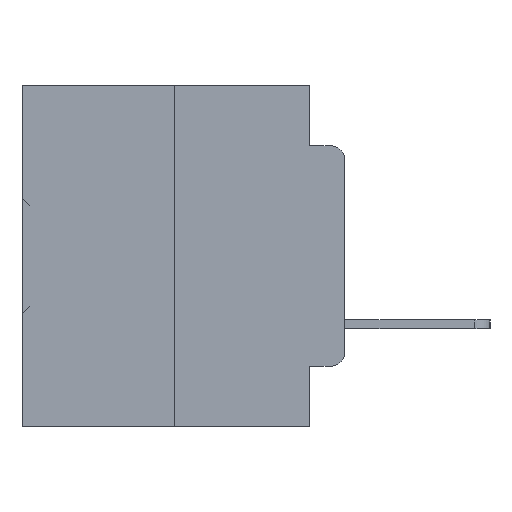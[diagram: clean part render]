
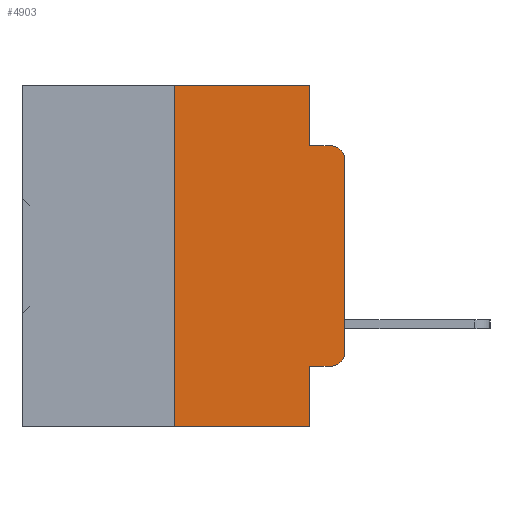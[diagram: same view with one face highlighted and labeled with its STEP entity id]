
A CAD part, left-side view. The second image highlights one B-rep face of the part: STEP entity #4903.
In plain terms, the highlighted planar face has unit normal (-1, 0, 0).
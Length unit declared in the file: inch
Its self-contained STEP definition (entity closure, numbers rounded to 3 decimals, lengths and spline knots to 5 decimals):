
#612 = DIRECTION ( 'NONE',  ( -1., 0., 0. ) ) ;
#797 = VERTEX_POINT ( 'NONE', #19545 ) ;
#963 = CIRCLE ( 'NONE', #14229, 0.02 ) ;
#1004 = CARTESIAN_POINT ( 'NONE',  ( 0., 0.051, -0.5 ) ) ;
#1061 = CARTESIAN_POINT ( 'NONE',  ( 0., 0.02, -0.1085 ) ) ;
#1221 = CARTESIAN_POINT ( 'NONE',  ( 0., 0.051, 0. ) ) ;
#2265 = LINE ( 'NONE', #32756, #8980 ) ;
#3630 = DIRECTION ( 'NONE',  ( 0., 0., 1. ) ) ;
#3919 = DIRECTION ( 'NONE',  ( 0., 0., -1. ) ) ;
#4000 = VECTOR ( 'NONE', #21444, 39.37008 ) ;
#4903 = ADVANCED_FACE ( 'NONE', ( #13401 ), #12431, .F. ) ;
#4946 = EDGE_CURVE ( 'NONE', #22276, #19420, #26978, .T. ) ;
#4949 = CARTESIAN_POINT ( 'NONE',  ( 0., 0.473, -0.5 ) ) ;
#5022 = LINE ( 'NONE', #25065, #19402 ) ;
#5251 = CARTESIAN_POINT ( 'NONE',  ( 0., 0.051, -0.0885 ) ) ;
#5256 = EDGE_CURVE ( 'NONE', #797, #22692, #16078, .T. ) ;
#6160 = VERTEX_POINT ( 'NONE', #10235 ) ;
#6634 = ORIENTED_EDGE ( 'NONE', *, *, #33833, .T. ) ;
#6826 = DIRECTION ( 'NONE',  ( 1., 0., 0. ) ) ;
#8473 = VECTOR ( 'NONE', #28571, 39.37008 ) ;
#8831 = AXIS2_PLACEMENT_3D ( 'NONE', #18241, #6826, #26962 ) ;
#8980 = VECTOR ( 'NONE', #30006, 39.37008 ) ;
#9675 = ORIENTED_EDGE ( 'NONE', *, *, #17428, .T. ) ;
#10235 = CARTESIAN_POINT ( 'NONE',  ( 0., 0.051, -0.4115 ) ) ;
#10378 = CARTESIAN_POINT ( 'NONE',  ( 0., 0.02, -0.0885 ) ) ;
#11265 = AXIS2_PLACEMENT_3D ( 'NONE', #17803, #612, #20729 ) ;
#11407 = EDGE_CURVE ( 'NONE', #19420, #12179, #963, .T. ) ;
#11985 = ORIENTED_EDGE ( 'NONE', *, *, #28319, .F. ) ;
#12179 = VERTEX_POINT ( 'NONE', #10378 ) ;
#12345 = ORIENTED_EDGE ( 'NONE', *, *, #30972, .F. ) ;
#12431 = PLANE ( 'NONE',  #8831 ) ;
#12539 = ORIENTED_EDGE ( 'NONE', *, *, #11407, .T. ) ;
#12823 = VECTOR ( 'NONE', #22512, 39.37008 ) ;
#13401 = FACE_OUTER_BOUND ( 'NONE', #13784, .T. ) ;
#13784 = EDGE_LOOP ( 'NONE', ( #15743, #12539, #16898, #11985, #29637, #19176, #6634, #12345, #9675, #26119 ) ) ;
#13962 = LINE ( 'NONE', #32434, #35150 ) ;
#14034 = CARTESIAN_POINT ( 'NONE',  ( 0., 0.473, 0. ) ) ;
#14229 = AXIS2_PLACEMENT_3D ( 'NONE', #1061, #21174, #3919 ) ;
#14534 = CARTESIAN_POINT ( 'NONE',  ( 0., 0., -0.1085 ) ) ;
#15743 = ORIENTED_EDGE ( 'NONE', *, *, #4946, .T. ) ;
#16078 = LINE ( 'NONE', #14034, #8473 ) ;
#16674 = EDGE_CURVE ( 'NONE', #17187, #797, #13962, .T. ) ;
#16898 = ORIENTED_EDGE ( 'NONE', *, *, #19856, .F. ) ;
#17187 = VERTEX_POINT ( 'NONE', #28906 ) ;
#17428 = EDGE_CURVE ( 'NONE', #6160, #22193, #2265, .T. ) ;
#17803 = CARTESIAN_POINT ( 'NONE',  ( 0., 0.02, -0.3915 ) ) ;
#17805 = VERTEX_POINT ( 'NONE', #25849 ) ;
#18241 = CARTESIAN_POINT ( 'NONE',  ( 0., 0.473, 0. ) ) ;
#18506 = CARTESIAN_POINT ( 'NONE',  ( 0., 0., 0. ) ) ;
#19007 = DIRECTION ( 'NONE',  ( 0., -1., 0. ) ) ;
#19176 = ORIENTED_EDGE ( 'NONE', *, *, #16674, .F. ) ;
#19402 = VECTOR ( 'NONE', #27949, 39.37008 ) ;
#19420 = VERTEX_POINT ( 'NONE', #14534 ) ;
#19545 = CARTESIAN_POINT ( 'NONE',  ( 0., 0.25, 0. ) ) ;
#19856 = EDGE_CURVE ( 'NONE', #17805, #12179, #20549, .T. ) ;
#20098 = EDGE_CURVE ( 'NONE', #22193, #22276, #20972, .T. ) ;
#20549 = LINE ( 'NONE', #5251, #12823 ) ;
#20729 = DIRECTION ( 'NONE',  ( 0., 0., -1. ) ) ;
#20972 = CIRCLE ( 'NONE', #11265, 0.02 ) ;
#21174 = DIRECTION ( 'NONE',  ( -1., 0., 0. ) ) ;
#21444 = DIRECTION ( 'NONE',  ( 0., 0., 1. ) ) ;
#22193 = VERTEX_POINT ( 'NONE', #27790 ) ;
#22276 = VERTEX_POINT ( 'NONE', #25272 ) ;
#22512 = DIRECTION ( 'NONE',  ( 0., -1., 0. ) ) ;
#22692 = VERTEX_POINT ( 'NONE', #1221 ) ;
#25065 = CARTESIAN_POINT ( 'NONE',  ( 0., 0.051, 0. ) ) ;
#25272 = CARTESIAN_POINT ( 'NONE',  ( 0., 0., -0.3915 ) ) ;
#25849 = CARTESIAN_POINT ( 'NONE',  ( 0., 0.051, -0.0885 ) ) ;
#26001 = VERTEX_POINT ( 'NONE', #1004 ) ;
#26119 = ORIENTED_EDGE ( 'NONE', *, *, #20098, .T. ) ;
#26962 = DIRECTION ( 'NONE',  ( 0., 0., -1. ) ) ;
#26978 = LINE ( 'NONE', #18506, #4000 ) ;
#27311 = VECTOR ( 'NONE', #19007, 39.37008 ) ;
#27790 = CARTESIAN_POINT ( 'NONE',  ( 0., 0.02, -0.4115 ) ) ;
#27949 = DIRECTION ( 'NONE',  ( 0., 0., -1. ) ) ;
#28319 = EDGE_CURVE ( 'NONE', #22692, #17805, #35695, .T. ) ;
#28571 = DIRECTION ( 'NONE',  ( 0., -1., 0. ) ) ;
#28680 = CARTESIAN_POINT ( 'NONE',  ( 0., 0.051, 0. ) ) ;
#28906 = CARTESIAN_POINT ( 'NONE',  ( 0., 0.25, -0.5 ) ) ;
#29637 = ORIENTED_EDGE ( 'NONE', *, *, #5256, .F. ) ;
#30006 = DIRECTION ( 'NONE',  ( 0., -1., 0. ) ) ;
#30972 = EDGE_CURVE ( 'NONE', #6160, #26001, #5022, .T. ) ;
#31557 = DIRECTION ( 'NONE',  ( 0., 0., -1. ) ) ;
#32434 = CARTESIAN_POINT ( 'NONE',  ( 0., 0.25, 0. ) ) ;
#32756 = CARTESIAN_POINT ( 'NONE',  ( 0., 0.051, -0.4115 ) ) ;
#33833 = EDGE_CURVE ( 'NONE', #17187, #26001, #34045, .T. ) ;
#34045 = LINE ( 'NONE', #4949, #27311 ) ;
#34809 = VECTOR ( 'NONE', #31557, 39.37008 ) ;
#35150 = VECTOR ( 'NONE', #3630, 39.37008 ) ;
#35695 = LINE ( 'NONE', #28680, #34809 ) ;
